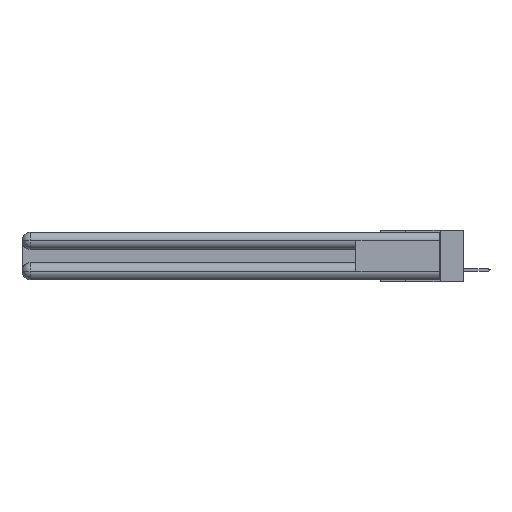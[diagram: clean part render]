
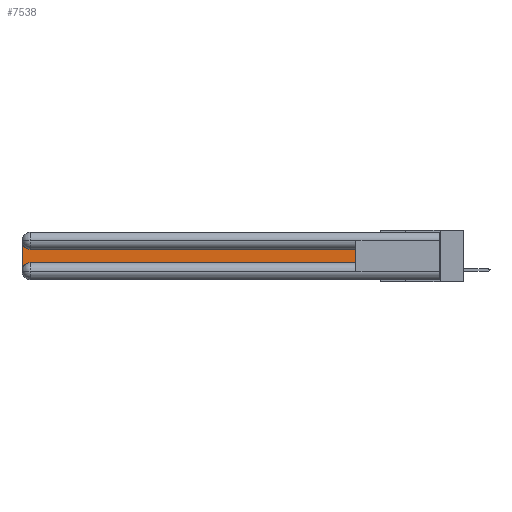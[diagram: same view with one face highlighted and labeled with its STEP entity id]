
A CAD part, left-side view. The second image highlights one B-rep face of the part: STEP entity #7538.
In plain terms, the highlighted planar face has unit normal (-1, 0, 0).
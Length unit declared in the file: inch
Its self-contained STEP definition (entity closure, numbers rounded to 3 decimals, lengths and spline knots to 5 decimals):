
#122 = CARTESIAN_POINT ( 'NONE',  ( 0.075, 0.6, -0.2175 ) ) ;
#187 = DIRECTION ( 'NONE',  ( 0., 0., -1. ) ) ;
#1014 = LINE ( 'NONE', #25176, #7360 ) ;
#1387 = VECTOR ( 'NONE', #28636, 39.37008 ) ;
#2207 = AXIS2_PLACEMENT_3D ( 'NONE', #28578, #19618, #12887 ) ;
#2885 = AXIS2_PLACEMENT_3D ( 'NONE', #9345, #25137, #187 ) ;
#3313 = VERTEX_POINT ( 'NONE', #4062 ) ;
#3378 = VERTEX_POINT ( 'NONE', #25167 ) ;
#3436 = LINE ( 'NONE', #122, #9813 ) ;
#4062 = CARTESIAN_POINT ( 'NONE',  ( 0.075, 3., -0.2775 ) ) ;
#4069 = EDGE_CURVE ( 'NONE', #3378, #12480, #10092, .T. ) ;
#4982 = CARTESIAN_POINT ( 'NONE',  ( 0.075, 2.94, -0.2175 ) ) ;
#5533 = AXIS2_PLACEMENT_3D ( 'NONE', #15675, #13391, #8934 ) ;
#5534 = ORIENTED_EDGE ( 'NONE', *, *, #14900, .T. ) ;
#7360 = VECTOR ( 'NONE', #20854, 39.37008 ) ;
#7511 = CARTESIAN_POINT ( 'NONE',  ( 0.075, 0.6, -0.1225 ) ) ;
#7538 = ADVANCED_FACE ( 'NONE', ( #22582 ), #21786, .F. ) ;
#8934 = DIRECTION ( 'NONE',  ( 0., 0., -1. ) ) ;
#9345 = CARTESIAN_POINT ( 'NONE',  ( 0.075, 2.94, -0.0625 ) ) ;
#9813 = VECTOR ( 'NONE', #27457, 39.37008 ) ;
#9999 = CARTESIAN_POINT ( 'NONE',  ( 0.075, 3., -0.0625 ) ) ;
#10092 = CIRCLE ( 'NONE', #2885, 0.06 ) ;
#10584 = LINE ( 'NONE', #19974, #1387 ) ;
#10852 = EDGE_LOOP ( 'NONE', ( #16869, #22748, #20352, #5534, #24161, #17927 ) ) ;
#11255 = CARTESIAN_POINT ( 'NONE',  ( 0.075, 0.6, -0.2175 ) ) ;
#11375 = LINE ( 'NONE', #18556, #15635 ) ;
#12480 = VERTEX_POINT ( 'NONE', #9999 ) ;
#12887 = DIRECTION ( 'NONE',  ( 0., 0., -1. ) ) ;
#13391 = DIRECTION ( 'NONE',  ( 1., 0., 0. ) ) ;
#13702 = DIRECTION ( 'NONE',  ( 0., 1., 0. ) ) ;
#14900 = EDGE_CURVE ( 'NONE', #3313, #15053, #21902, .T. ) ;
#15053 = VERTEX_POINT ( 'NONE', #4982 ) ;
#15635 = VECTOR ( 'NONE', #13702, 39.37008 ) ;
#15675 = CARTESIAN_POINT ( 'NONE',  ( 0.075, 2.94, -0.2775 ) ) ;
#16869 = ORIENTED_EDGE ( 'NONE', *, *, #19472, .T. ) ;
#17927 = ORIENTED_EDGE ( 'NONE', *, *, #21298, .T. ) ;
#18556 = CARTESIAN_POINT ( 'NONE',  ( 0.075, 0.6, -0.1225 ) ) ;
#19472 = EDGE_CURVE ( 'NONE', #21424, #3378, #11375, .T. ) ;
#19618 = DIRECTION ( 'NONE',  ( 1., 0., 0. ) ) ;
#19974 = CARTESIAN_POINT ( 'NONE',  ( 0.075, 3., -0.2175 ) ) ;
#20352 = ORIENTED_EDGE ( 'NONE', *, *, #20946, .T. ) ;
#20854 = DIRECTION ( 'NONE',  ( 0., 0., 1. ) ) ;
#20946 = EDGE_CURVE ( 'NONE', #12480, #3313, #10584, .T. ) ;
#21298 = EDGE_CURVE ( 'NONE', #27712, #21424, #1014, .T. ) ;
#21424 = VERTEX_POINT ( 'NONE', #7511 ) ;
#21786 = PLANE ( 'NONE',  #2207 ) ;
#21902 = CIRCLE ( 'NONE', #5533, 0.06 ) ;
#22582 = FACE_OUTER_BOUND ( 'NONE', #10852, .T. ) ;
#22748 = ORIENTED_EDGE ( 'NONE', *, *, #4069, .T. ) ;
#24161 = ORIENTED_EDGE ( 'NONE', *, *, #24333, .T. ) ;
#24333 = EDGE_CURVE ( 'NONE', #15053, #27712, #3436, .T. ) ;
#25137 = DIRECTION ( 'NONE',  ( 1., 0., 0. ) ) ;
#25167 = CARTESIAN_POINT ( 'NONE',  ( 0.075, 2.94, -0.1225 ) ) ;
#25176 = CARTESIAN_POINT ( 'NONE',  ( 0.075, 0.6, -0.2175 ) ) ;
#27457 = DIRECTION ( 'NONE',  ( 0., -1., 0. ) ) ;
#27712 = VERTEX_POINT ( 'NONE', #11255 ) ;
#28578 = CARTESIAN_POINT ( 'NONE',  ( 0.075, 3., -0.1225 ) ) ;
#28636 = DIRECTION ( 'NONE',  ( 0., 0., -1. ) ) ;
